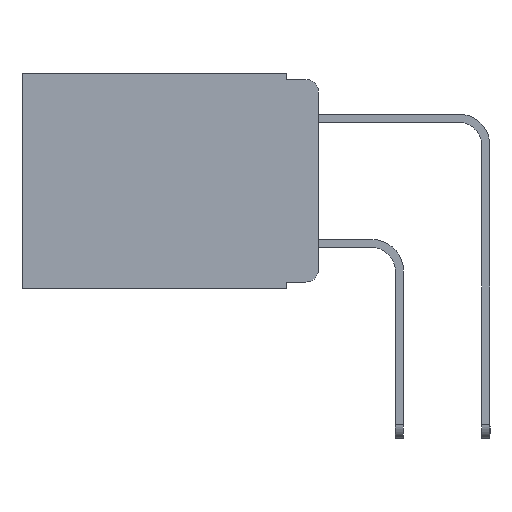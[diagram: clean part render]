
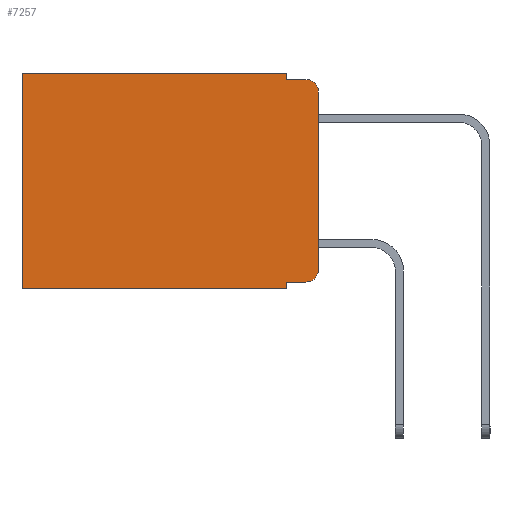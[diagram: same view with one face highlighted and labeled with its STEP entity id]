
A CAD part, left-side view. The second image highlights one B-rep face of the part: STEP entity #7257.
In plain terms, the highlighted planar face has unit normal (-1, 0, 0).
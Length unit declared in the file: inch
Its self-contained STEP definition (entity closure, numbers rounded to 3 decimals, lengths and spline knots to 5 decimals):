
#174 = CARTESIAN_POINT ( 'NONE',  ( 0.298, 0.473, 0. ) ) ;
#435 = VECTOR ( 'NONE', #23152, 39.37008 ) ;
#538 = PLANE ( 'NONE',  #14729 ) ;
#844 = DIRECTION ( 'NONE',  ( 0., -1., 0. ) ) ;
#922 = LINE ( 'NONE', #8104, #5009 ) ;
#1202 = CARTESIAN_POINT ( 'NONE',  ( 0.298, 0., 0. ) ) ;
#1791 = DIRECTION ( 'NONE',  ( 0., 1., 0. ) ) ;
#1818 = CARTESIAN_POINT ( 'NONE',  ( 0.298, 0.051, -0.333 ) ) ;
#2054 = ORIENTED_EDGE ( 'NONE', *, *, #22742, .T. ) ;
#2083 = EDGE_CURVE ( 'NONE', #12338, #12870, #922, .T. ) ;
#2286 = CARTESIAN_POINT ( 'NONE',  ( 0.298, 0.02, -0.03 ) ) ;
#2758 = EDGE_CURVE ( 'NONE', #12336, #10779, #7399, .T. ) ;
#3045 = CARTESIAN_POINT ( 'NONE',  ( 0.298, 0.051, -0.343 ) ) ;
#3479 = VERTEX_POINT ( 'NONE', #15103 ) ;
#3525 = AXIS2_PLACEMENT_3D ( 'NONE', #8564, #17491, #4682 ) ;
#3560 = LINE ( 'NONE', #8970, #16529 ) ;
#3891 = VECTOR ( 'NONE', #21735, 39.37008 ) ;
#4031 = DIRECTION ( 'NONE',  ( -1., 0., 0. ) ) ;
#4255 = CARTESIAN_POINT ( 'NONE',  ( 0.298, 0.051, -0.01 ) ) ;
#4370 = LINE ( 'NONE', #4255, #17087 ) ;
#4532 = CARTESIAN_POINT ( 'NONE',  ( 0.298, 0.473, 0. ) ) ;
#4682 = DIRECTION ( 'NONE',  ( 0., 0., -1. ) ) ;
#4802 = EDGE_CURVE ( 'NONE', #8690, #12870, #17333, .T. ) ;
#5009 = VECTOR ( 'NONE', #9638, 39.37008 ) ;
#5139 = CARTESIAN_POINT ( 'NONE',  ( 0.298, 0.051, 0. ) ) ;
#5423 = DIRECTION ( 'NONE',  ( 0., 0., -1. ) ) ;
#5483 = CARTESIAN_POINT ( 'NONE',  ( 0.298, 0., 0. ) ) ;
#5530 = AXIS2_PLACEMENT_3D ( 'NONE', #2286, #4031, #21907 ) ;
#6498 = VERTEX_POINT ( 'NONE', #17499 ) ;
#6949 = EDGE_LOOP ( 'NONE', ( #13851, #16429, #13627, #15494, #20161, #22144, #16358, #10829, #2054, #10634 ) ) ;
#7257 = ADVANCED_FACE ( 'NONE', ( #8055 ), #538, .F. ) ;
#7399 = LINE ( 'NONE', #5139, #3891 ) ;
#7646 = CARTESIAN_POINT ( 'NONE',  ( 0.298, 0., -0.03 ) ) ;
#8055 = FACE_OUTER_BOUND ( 'NONE', #6949, .T. ) ;
#8104 = CARTESIAN_POINT ( 'NONE',  ( 0.298, 0., -0.343 ) ) ;
#8382 = LINE ( 'NONE', #1202, #17999 ) ;
#8564 = CARTESIAN_POINT ( 'NONE',  ( 0.298, 0.02, -0.313 ) ) ;
#8690 = VERTEX_POINT ( 'NONE', #174 ) ;
#8826 = LINE ( 'NONE', #9183, #435 ) ;
#8970 = CARTESIAN_POINT ( 'NONE',  ( 0.298, 0.051, 0. ) ) ;
#9183 = CARTESIAN_POINT ( 'NONE',  ( 0.298, 0.051, -0.333 ) ) ;
#9638 = DIRECTION ( 'NONE',  ( 0., 1., 0. ) ) ;
#9648 = CIRCLE ( 'NONE', #5530, 0.02 ) ;
#9835 = VERTEX_POINT ( 'NONE', #7646 ) ;
#9929 = DIRECTION ( 'NONE',  ( 1., 0., 0. ) ) ;
#10144 = EDGE_CURVE ( 'NONE', #9835, #6498, #17599, .T. ) ;
#10634 = ORIENTED_EDGE ( 'NONE', *, *, #12283, .T. ) ;
#10779 = VERTEX_POINT ( 'NONE', #22221 ) ;
#10829 = ORIENTED_EDGE ( 'NONE', *, *, #19584, .F. ) ;
#12283 = EDGE_CURVE ( 'NONE', #15643, #6498, #18907, .T. ) ;
#12301 = DIRECTION ( 'NONE',  ( 0., 0., -1. ) ) ;
#12336 = VERTEX_POINT ( 'NONE', #22445 ) ;
#12338 = VERTEX_POINT ( 'NONE', #3045 ) ;
#12870 = VERTEX_POINT ( 'NONE', #22983 ) ;
#13443 = EDGE_CURVE ( 'NONE', #10779, #3479, #4370, .T. ) ;
#13627 = ORIENTED_EDGE ( 'NONE', *, *, #13443, .F. ) ;
#13851 = ORIENTED_EDGE ( 'NONE', *, *, #10144, .F. ) ;
#13911 = DIRECTION ( 'NONE',  ( 0., 0., -1. ) ) ;
#14729 = AXIS2_PLACEMENT_3D ( 'NONE', #18861, #9929, #18403 ) ;
#15006 = VECTOR ( 'NONE', #13911, 39.37008 ) ;
#15103 = CARTESIAN_POINT ( 'NONE',  ( 0.298, 0.02, -0.01 ) ) ;
#15411 = EDGE_CURVE ( 'NONE', #9835, #3479, #9648, .T. ) ;
#15494 = ORIENTED_EDGE ( 'NONE', *, *, #2758, .F. ) ;
#15643 = VERTEX_POINT ( 'NONE', #22824 ) ;
#16358 = ORIENTED_EDGE ( 'NONE', *, *, #2083, .F. ) ;
#16429 = ORIENTED_EDGE ( 'NONE', *, *, #15411, .T. ) ;
#16529 = VECTOR ( 'NONE', #5423, 39.37008 ) ;
#17087 = VECTOR ( 'NONE', #844, 39.37008 ) ;
#17247 = VERTEX_POINT ( 'NONE', #1818 ) ;
#17333 = LINE ( 'NONE', #4532, #15006 ) ;
#17491 = DIRECTION ( 'NONE',  ( -1., 0., 0. ) ) ;
#17499 = CARTESIAN_POINT ( 'NONE',  ( 0.298, 0., -0.313 ) ) ;
#17599 = LINE ( 'NONE', #5483, #18951 ) ;
#17999 = VECTOR ( 'NONE', #1791, 39.37008 ) ;
#18403 = DIRECTION ( 'NONE',  ( 0., 0., -1. ) ) ;
#18861 = CARTESIAN_POINT ( 'NONE',  ( 0.298, 0., 0. ) ) ;
#18907 = CIRCLE ( 'NONE', #3525, 0.02 ) ;
#18951 = VECTOR ( 'NONE', #12301, 39.37008 ) ;
#19544 = EDGE_CURVE ( 'NONE', #12336, #8690, #8382, .T. ) ;
#19584 = EDGE_CURVE ( 'NONE', #17247, #12338, #3560, .T. ) ;
#20161 = ORIENTED_EDGE ( 'NONE', *, *, #19544, .T. ) ;
#21735 = DIRECTION ( 'NONE',  ( 0., 0., -1. ) ) ;
#21907 = DIRECTION ( 'NONE',  ( 0., 0., -1. ) ) ;
#22144 = ORIENTED_EDGE ( 'NONE', *, *, #4802, .T. ) ;
#22221 = CARTESIAN_POINT ( 'NONE',  ( 0.298, 0.051, -0.01 ) ) ;
#22445 = CARTESIAN_POINT ( 'NONE',  ( 0.298, 0.051, 0. ) ) ;
#22742 = EDGE_CURVE ( 'NONE', #17247, #15643, #8826, .T. ) ;
#22824 = CARTESIAN_POINT ( 'NONE',  ( 0.298, 0.02, -0.333 ) ) ;
#22983 = CARTESIAN_POINT ( 'NONE',  ( 0.298, 0.473, -0.343 ) ) ;
#23152 = DIRECTION ( 'NONE',  ( 0., -1., 0. ) ) ;
